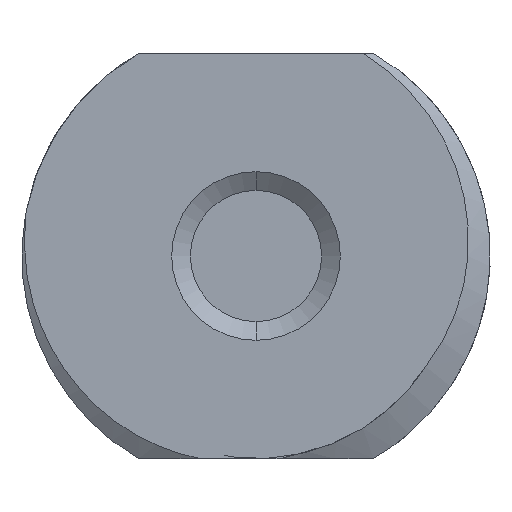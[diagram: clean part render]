
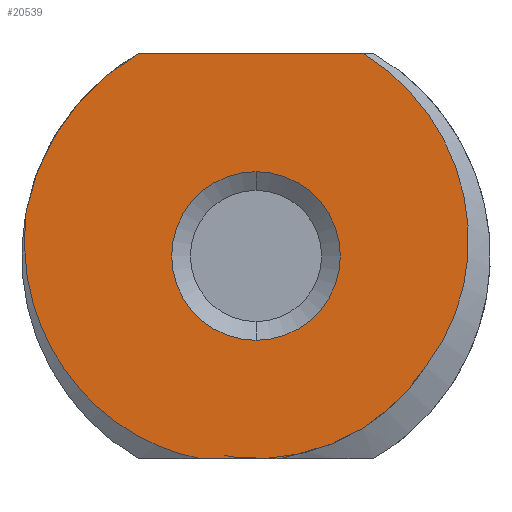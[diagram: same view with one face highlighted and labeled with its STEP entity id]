
A CAD part, left-side view. The second image highlights one B-rep face of the part: STEP entity #20539.
In plain terms, the highlighted planar face has unit normal (-1, 0, 0).
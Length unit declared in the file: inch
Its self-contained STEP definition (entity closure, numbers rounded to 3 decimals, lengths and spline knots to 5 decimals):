
#619 = ORIENTED_EDGE ( 'NONE', *, *, #9826, .T. ) ;
#759 = CIRCLE ( 'NONE', #12928, 0.045 ) ;
#778 = CARTESIAN_POINT ( 'NONE',  ( 0.1425, -0.88321, 0.10238 ) ) ;
#847 = CARTESIAN_POINT ( 'NONE',  ( 0.1425, -1.007, 0.1081 ) ) ;
#893 = CARTESIAN_POINT ( 'NONE',  ( 0.1425, -1.007, 0.1081 ) ) ;
#1809 = ORIENTED_EDGE ( 'NONE', *, *, #7828, .T. ) ;
#1989 = CARTESIAN_POINT ( 'NONE',  ( 0.1425, -1.09756, 0.0491 ) ) ;
#2250 = FACE_BOUND ( 'NONE', #3519, .T. ) ;
#2383 = CARTESIAN_POINT ( 'NONE',  ( 0.1425, -0.94902, 0.00916 ) ) ;
#2454 = CARTESIAN_POINT ( 'NONE',  ( 0.1425, -1.07123, 0.21192 ) ) ;
#2523 = CARTESIAN_POINT ( 'NONE',  ( 0.1425, -0.91381, 0.03588 ) ) ;
#2622 = DIRECTION ( 'NONE',  ( 1., 0., 0. ) ) ;
#2957 = VERTEX_POINT ( 'NONE', #18040 ) ;
#3076 = VERTEX_POINT ( 'NONE', #16622 ) ;
#3191 = CARTESIAN_POINT ( 'NONE',  ( 0.1425, -1.07394, 0.02294 ) ) ;
#3301 = VERTEX_POINT ( 'NONE', #6522 ) ;
#3519 = EDGE_LOOP ( 'NONE', ( #17458, #20648 ) ) ;
#3552 = CARTESIAN_POINT ( 'NONE',  ( 0.1425, -1.007, 0. ) ) ;
#3739 = CARTESIAN_POINT ( 'NONE',  ( 0.1425, -1.10249, 0.05549 ) ) ;
#4005 = EDGE_CURVE ( 'NONE', #11370, #3076, #12005, .T. ) ;
#4012 = CARTESIAN_POINT ( 'NONE',  ( 0.1425, -1.11603, 0.08443 ) ) ;
#4151 = VERTEX_POINT ( 'NONE', #7479 ) ;
#4175 = DIRECTION ( 'NONE',  ( 0., 0., -1. ) ) ;
#4304 = ORIENTED_EDGE ( 'NONE', *, *, #4005, .T. ) ;
#4861 = LINE ( 'NONE', #3552, #8646 ) ;
#4992 = AXIS2_PLACEMENT_3D ( 'NONE', #847, #5838, #15257 ) ;
#5284 = ORIENTED_EDGE ( 'NONE', *, *, #8225, .T. ) ;
#5351 = CARTESIAN_POINT ( 'NONE',  ( 0.1425, -1.09368, 0.04314 ) ) ;
#5357 = CARTESIAN_POINT ( 'NONE',  ( 0.1425, -1.1195, 0.1 ) ) ;
#5464 = ORIENTED_EDGE ( 'NONE', *, *, #7253, .T. ) ;
#5512 = ORIENTED_EDGE ( 'NONE', *, *, #7137, .F. ) ;
#5620 = CARTESIAN_POINT ( 'NONE',  ( 0.1425, -1.10664, 0.06229 ) ) ;
#5687 = CARTESIAN_POINT ( 'NONE',  ( 0.1425, -0.97718, 0. ) ) ;
#5762 = CARTESIAN_POINT ( 'NONE',  ( 0.1425, -0.89689, 0.06024 ) ) ;
#5838 = DIRECTION ( 'NONE',  ( 1., 0., 0. ) ) ;
#6522 = CARTESIAN_POINT ( 'NONE',  ( 0.1425, -0.97718, 0. ) ) ;
#7137 = EDGE_CURVE ( 'NONE', #2957, #15188, #14432, .T. ) ;
#7145 = ORIENTED_EDGE ( 'NONE', *, *, #19283, .T. ) ;
#7250 = DIRECTION ( 'NONE',  ( 0., 0., -1. ) ) ;
#7253 = EDGE_CURVE ( 'NONE', #2957, #3301, #7567, .T. ) ;
#7256 = CARTESIAN_POINT ( 'NONE',  ( 0.1425, -0.92433, 0.02553 ) ) ;
#7260 = CARTESIAN_POINT ( 'NONE',  ( 0.1425, -1.11643, 0.14759 ) ) ;
#7327 = CARTESIAN_POINT ( 'NONE',  ( 0.1425, -0.88247, 0.11717 ) ) ;
#7479 = CARTESIAN_POINT ( 'NONE',  ( 0.1425, -1.01983, 0. ) ) ;
#7495 = CARTESIAN_POINT ( 'NONE',  ( 0.1425, -1.007, 0.1081 ) ) ;
#7546 = CARTESIAN_POINT ( 'NONE',  ( 0.1425, -1.10374, 0.17693 ) ) ;
#7567 = B_SPLINE_CURVE_WITH_KNOTS ( 'NONE', 3,
 ( #16947, #7327, #778, #12044, #20205, #5762, #10486, #18644, #2523, #7256, #10558, #12183, #2383, #9009, #13784, #5687 ),
 .UNSPECIFIED., .F., .F.,
 ( 4, 2, 2, 2, 2, 2, 2, 4 ),
 ( 0., 0.00112, 0.00168, 0.00224, 0.00281, 0.00337, 0.00393, 0.00449 ),
 .UNSPECIFIED. ) ;
#7807 = FACE_OUTER_BOUND ( 'NONE', #16630, .T. ) ;
#7828 = EDGE_CURVE ( 'NONE', #4151, #16165, #10943, .T. ) ;
#8161 = VECTOR ( 'NONE', #17115, 39.37008 ) ;
#8225 = EDGE_CURVE ( 'NONE', #3301, #4151, #4861, .T. ) ;
#8258 = CARTESIAN_POINT ( 'NONE',  ( 0.1425, -1.007, 0.1531 ) ) ;
#8612 = CARTESIAN_POINT ( 'NONE',  ( 0.1425, -1.12043, 0.12401 ) ) ;
#8646 = VECTOR ( 'NONE', #14806, 39.37008 ) ;
#8871 = LINE ( 'NONE', #13731, #8161 ) ;
#9009 = CARTESIAN_POINT ( 'NONE',  ( 0.1425, -0.9627, 0.00356 ) ) ;
#9110 = CARTESIAN_POINT ( 'NONE',  ( 0.1425, -1.02932, 0.00234 ) ) ;
#9235 = CARTESIAN_POINT ( 'NONE',  ( 0.1425, -1.08917, 0.19609 ) ) ;
#9303 = CARTESIAN_POINT ( 'NONE',  ( 0.1425, -1.02302, 0.00063 ) ) ;
#9603 = CARTESIAN_POINT ( 'NONE',  ( 0.1425, -1.05639, 0.01092 ) ) ;
#9826 = EDGE_CURVE ( 'NONE', #3076, #15188, #8871, .T. ) ;
#9904 = B_SPLINE_CURVE_WITH_KNOTS ( 'NONE', 3,
 ( #15996, #19250, #9603, #3191, #17679, #10078, #5351, #1989 ),
 .UNSPECIFIED., .F., .F.,
 ( 4, 2, 2, 4 ),
 ( 0., 0.00108, 0.00163, 0.00217 ),
 .UNSPECIFIED. ) ;
#10078 = CARTESIAN_POINT ( 'NONE',  ( 0.1425, -1.0892, 0.03756 ) ) ;
#10486 = CARTESIAN_POINT ( 'NONE',  ( 0.1425, -0.90056, 0.05373 ) ) ;
#10558 = CARTESIAN_POINT ( 'NONE',  ( 0.1425, -0.93016, 0.02077 ) ) ;
#10638 = CARTESIAN_POINT ( 'NONE',  ( 0.1425, -1.07758, 0.20701 ) ) ;
#10776 = CARTESIAN_POINT ( 'NONE',  ( 0.1425, -1.02932, 0.00234 ) ) ;
#10943 = B_SPLINE_CURVE_WITH_KNOTS ( 'NONE', 3,
 ( #10991, #9303, #18790, #10776 ),
 .UNSPECIFIED., .F., .F.,
 ( 4, 4 ),
 ( 0.00557, 0.00582 ),
 .UNSPECIFIED. ) ;
#10991 = CARTESIAN_POINT ( 'NONE',  ( 0.1425, -1.01983, 0. ) ) ;
#11123 = VERTEX_POINT ( 'NONE', #8258 ) ;
#11370 = VERTEX_POINT ( 'NONE', #16220 ) ;
#11779 = CARTESIAN_POINT ( 'NONE',  ( 0.1425, -1.11399, 0.15534 ) ) ;
#12005 = B_SPLINE_CURVE_WITH_KNOTS ( 'NONE', 3,
 ( #16809, #3739, #5620, #13644, #4012, #5357, #15260, #8612, #16880, #7260, #11779, #20489, #7546, #18794, #9235, #10638, #2454, #15630 ),
 .UNSPECIFIED., .F., .F.,
 ( 4, 2, 2, 2, 2, 2, 2, 2, 4 ),
 ( 0., 0.00061, 0.00121, 0.00182, 0.00243, 0.00303, 0.00364, 0.00424, 0.00485 ),
 .UNSPECIFIED. ) ;
#12044 = CARTESIAN_POINT ( 'NONE',  ( 0.1425, -0.88846, 0.08064 ) ) ;
#12183 = CARTESIAN_POINT ( 'NONE',  ( 0.1425, -0.94251, 0.0126 ) ) ;
#12223 = CARTESIAN_POINT ( 'NONE',  ( 0.1425, -1.007, 0.0631 ) ) ;
#12234 = DIRECTION ( 'NONE',  ( 1., 0., 0. ) ) ;
#12928 = AXIS2_PLACEMENT_3D ( 'NONE', #15621, #15321, #7250 ) ;
#13644 = CARTESIAN_POINT ( 'NONE',  ( 0.1425, -1.1134, 0.07672 ) ) ;
#13731 = CARTESIAN_POINT ( 'NONE',  ( 0.1425, -1.007, 0.21619 ) ) ;
#13784 = CARTESIAN_POINT ( 'NONE',  ( 0.1425, -0.96993, 0.0014 ) ) ;
#14113 = AXIS2_PLACEMENT_3D ( 'NONE', #7495, #2622, #4175 ) ;
#14432 = CIRCLE ( 'NONE', #4992, 0.125 ) ;
#14544 = VERTEX_POINT ( 'NONE', #12223 ) ;
#14806 = DIRECTION ( 'NONE',  ( 0., -1., 0. ) ) ;
#15188 = VERTEX_POINT ( 'NONE', #15871 ) ;
#15257 = DIRECTION ( 'NONE',  ( 0., 0., -1. ) ) ;
#15260 = CARTESIAN_POINT ( 'NONE',  ( 0.1425, -1.12036, 0.10792 ) ) ;
#15321 = DIRECTION ( 'NONE',  ( 1., 0., 0. ) ) ;
#15621 = CARTESIAN_POINT ( 'NONE',  ( 0.1425, -1.007, 0.1081 ) ) ;
#15630 = CARTESIAN_POINT ( 'NONE',  ( 0.1425, -1.06442, 0.21619 ) ) ;
#15871 = CARTESIAN_POINT ( 'NONE',  ( 0.1425, -0.94422, 0.21619 ) ) ;
#15996 = CARTESIAN_POINT ( 'NONE',  ( 0.1425, -1.02932, 0.00234 ) ) ;
#16165 = VERTEX_POINT ( 'NONE', #9110 ) ;
#16180 = EDGE_CURVE ( 'NONE', #14544, #11123, #20146, .T. ) ;
#16220 = CARTESIAN_POINT ( 'NONE',  ( 0.1425, -1.09756, 0.0491 ) ) ;
#16622 = CARTESIAN_POINT ( 'NONE',  ( 0.1425, -1.06442, 0.21619 ) ) ;
#16630 = EDGE_LOOP ( 'NONE', ( #4304, #619, #5512, #5464, #5284, #1809, #7145 ) ) ;
#16809 = CARTESIAN_POINT ( 'NONE',  ( 0.1425, -1.09756, 0.0491 ) ) ;
#16880 = CARTESIAN_POINT ( 'NONE',  ( 0.1425, -1.11963, 0.13199 ) ) ;
#16947 = CARTESIAN_POINT ( 'NONE',  ( 0.1425, -0.88431, 0.132 ) ) ;
#17115 = DIRECTION ( 'NONE',  ( 0., 1., 0. ) ) ;
#17225 = EDGE_CURVE ( 'NONE', #11123, #14544, #759, .T. ) ;
#17458 = ORIENTED_EDGE ( 'NONE', *, *, #17225, .T. ) ;
#17679 = CARTESIAN_POINT ( 'NONE',  ( 0.1425, -1.07933, 0.02747 ) ) ;
#18040 = CARTESIAN_POINT ( 'NONE',  ( 0.1425, -0.88431, 0.132 ) ) ;
#18619 = DIRECTION ( 'NONE',  ( 0., 0., -1. ) ) ;
#18644 = CARTESIAN_POINT ( 'NONE',  ( 0.1425, -0.90906, 0.04152 ) ) ;
#18790 = CARTESIAN_POINT ( 'NONE',  ( 0.1425, -1.02618, 0.00141 ) ) ;
#18794 = CARTESIAN_POINT ( 'NONE',  ( 0.1425, -1.09451, 0.19 ) ) ;
#19250 = CARTESIAN_POINT ( 'NONE',  ( 0.1425, -1.04324, 0.00528 ) ) ;
#19283 = EDGE_CURVE ( 'NONE', #16165, #11370, #9904, .T. ) ;
#20146 = CIRCLE ( 'NONE', #14113, 0.045 ) ;
#20181 = PLANE ( 'NONE',  #20569 ) ;
#20205 = CARTESIAN_POINT ( 'NONE',  ( 0.1425, -0.89085, 0.07367 ) ) ;
#20489 = CARTESIAN_POINT ( 'NONE',  ( 0.1425, -1.10764, 0.16999 ) ) ;
#20539 = ADVANCED_FACE ( 'NONE', ( #2250, #7807 ), #20181, .F. ) ;
#20569 = AXIS2_PLACEMENT_3D ( 'NONE', #893, #12234, #18619 ) ;
#20648 = ORIENTED_EDGE ( 'NONE', *, *, #16180, .T. ) ;
